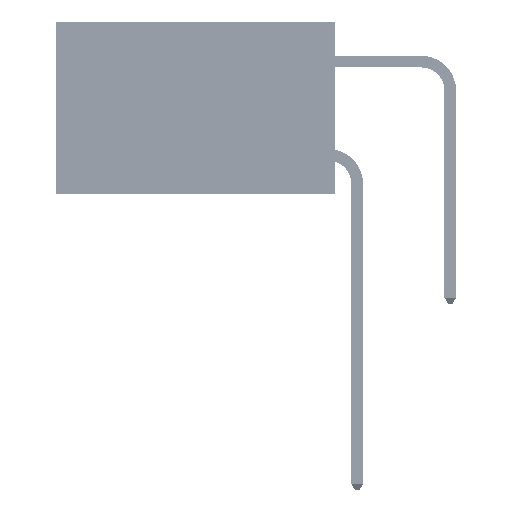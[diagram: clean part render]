
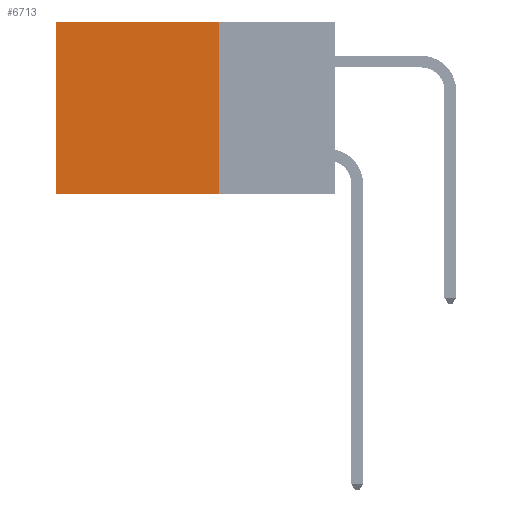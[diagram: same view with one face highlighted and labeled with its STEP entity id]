
A CAD part, left-side view. The second image highlights one B-rep face of the part: STEP entity #6713.
In plain terms, the highlighted planar face has unit normal (-1, 0, 0).
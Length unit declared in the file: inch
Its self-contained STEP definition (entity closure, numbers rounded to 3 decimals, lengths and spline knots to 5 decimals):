
#831 = LINE ( 'NONE', #17465, #1989 ) ;
#1543 = EDGE_LOOP ( 'NONE', ( #43137, #11822, #22316, #41230 ) ) ;
#1989 = VECTOR ( 'NONE', #30015, 39.37008 ) ;
#2458 = DIRECTION ( 'NONE',  ( 0., 1., 0. ) ) ;
#2540 = VECTOR ( 'NONE', #6783, 39.37008 ) ;
#2961 = VERTEX_POINT ( 'NONE', #44906 ) ;
#3130 = EDGE_CURVE ( 'NONE', #16658, #8471, #39844, .T. ) ;
#5716 = LINE ( 'NONE', #43122, #2540 ) ;
#5886 = EDGE_CURVE ( 'NONE', #16658, #2961, #43830, .T. ) ;
#6031 = CARTESIAN_POINT ( 'NONE',  ( 0.2875, 0.25, 0. ) ) ;
#6247 = FACE_OUTER_BOUND ( 'NONE', #1543, .T. ) ;
#6493 = VECTOR ( 'NONE', #27177, 39.37008 ) ;
#6713 = ADVANCED_FACE ( 'NONE', ( #6247 ), #48284, .F. ) ;
#6783 = DIRECTION ( 'NONE',  ( 0., 0., -1. ) ) ;
#8471 = VERTEX_POINT ( 'NONE', #29449 ) ;
#11822 = ORIENTED_EDGE ( 'NONE', *, *, #41132, .F. ) ;
#15983 = VERTEX_POINT ( 'NONE', #26908 ) ;
#16658 = VERTEX_POINT ( 'NONE', #24791 ) ;
#17465 = CARTESIAN_POINT ( 'NONE',  ( 0.2875, 0.25, -0.37 ) ) ;
#21761 = VECTOR ( 'NONE', #2458, 39.37008 ) ;
#22316 = ORIENTED_EDGE ( 'NONE', *, *, #5886, .F. ) ;
#24791 = CARTESIAN_POINT ( 'NONE',  ( 0.2875, 0.25, 0. ) ) ;
#26908 = CARTESIAN_POINT ( 'NONE',  ( 0.2875, 0.6, -0.37 ) ) ;
#27177 = DIRECTION ( 'NONE',  ( 0., 0., -1. ) ) ;
#28327 = AXIS2_PLACEMENT_3D ( 'NONE', #31855, #44169, #39258 ) ;
#29449 = CARTESIAN_POINT ( 'NONE',  ( 0.2875, 0.6, 0. ) ) ;
#30015 = DIRECTION ( 'NONE',  ( 0., 1., 0. ) ) ;
#31855 = CARTESIAN_POINT ( 'NONE',  ( 0.2875, 0.25, 0. ) ) ;
#34592 = EDGE_CURVE ( 'NONE', #8471, #15983, #5716, .T. ) ;
#39258 = DIRECTION ( 'NONE',  ( 0., 0., -1. ) ) ;
#39844 = LINE ( 'NONE', #6031, #21761 ) ;
#41132 = EDGE_CURVE ( 'NONE', #2961, #15983, #831, .T. ) ;
#41230 = ORIENTED_EDGE ( 'NONE', *, *, #3130, .T. ) ;
#43031 = CARTESIAN_POINT ( 'NONE',  ( 0.2875, 0.25, 0. ) ) ;
#43122 = CARTESIAN_POINT ( 'NONE',  ( 0.2875, 0.6, 0. ) ) ;
#43137 = ORIENTED_EDGE ( 'NONE', *, *, #34592, .T. ) ;
#43830 = LINE ( 'NONE', #43031, #6493 ) ;
#44169 = DIRECTION ( 'NONE',  ( 1., 0., 0. ) ) ;
#44906 = CARTESIAN_POINT ( 'NONE',  ( 0.2875, 0.25, -0.37 ) ) ;
#48284 = PLANE ( 'NONE',  #28327 ) ;
